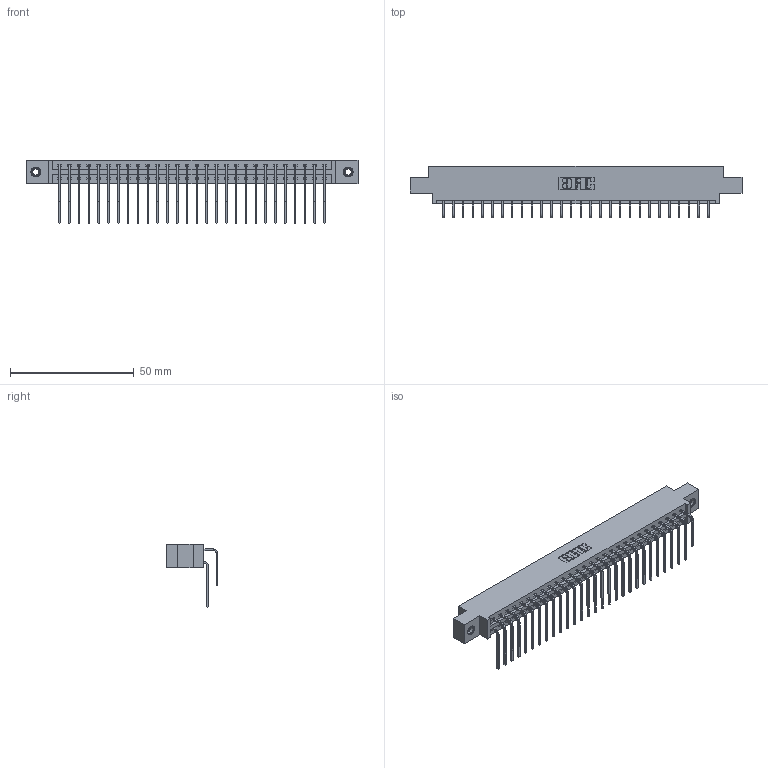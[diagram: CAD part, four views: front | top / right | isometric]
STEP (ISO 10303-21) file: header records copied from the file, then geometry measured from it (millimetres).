
FILE_DESCRIPTION (( 'STEP AP203' ), '1' );
FILE_NAME ('337-056-559-807.STEP', '2019-10-11T20:14:15', ( '' ), ( '' ), 'SwSTEP 2.0', 'SolidWorks 2016', '' );
FILE_SCHEMA (( 'CONFIG_CONTROL_DESIGN' ));
Length unit declared in the file: inch
Products named in the file (5): 345-292-001_559 Tail - 2; 345-250-001_345-250-005-103; 345-292-001_558 559 Tail - 1; 337-056-559-807; 337 Part_0.170 Offset - 0.156 Dia-TI
Assembly tree (59 placements, depth 2):
  337-056-559-807
    337 Part_0.170 Offset - 0.156 Dia-TI
    345-292-001_558 559 Tail - 1  x28
    345-292-001_559 Tail - 2  x28
    345-250-001_345-250-005-103  x2
Bounding box: 133.96 x 20.9 x 25.53 mm (x, y, z)
Volume: 14123.4 mm3; surface area: 17596.4 mm2
Topology: 59 solids, 59 shells, 3314 faces, 9811 edges, 6458 vertices
Faces by surface type: plane 2346, cylinder 952, cone 12, torus 4
Entity records: 26622 total; most frequent: CARTESIAN_POINT 4524, ORIENTED_EDGE 4402, DIRECTION 3887, EDGE_CURVE 2201, VECTOR 2013, LINE 2013, VERTEX_POINT 1460, AXIS2_PLACEMENT_3D 937
